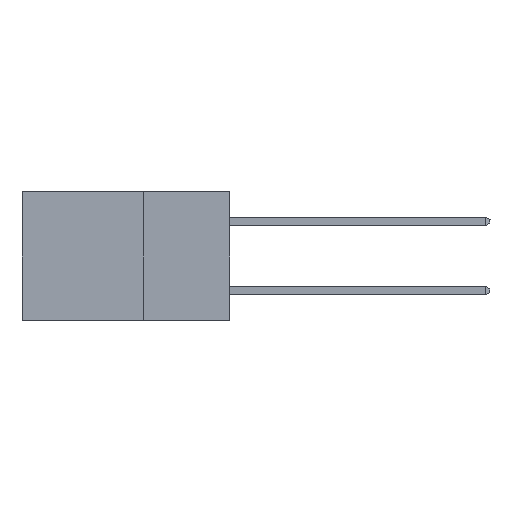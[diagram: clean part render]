
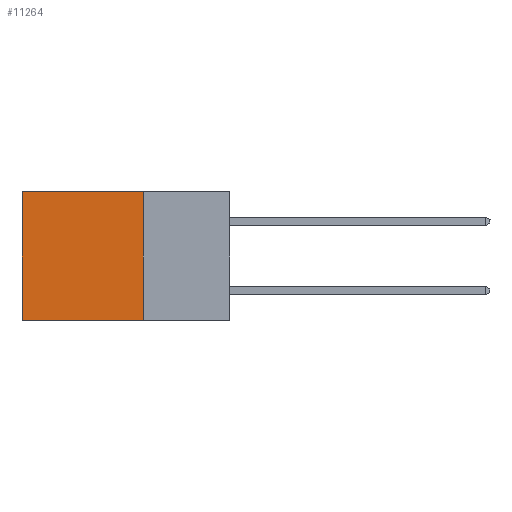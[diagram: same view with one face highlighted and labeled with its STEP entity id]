
A CAD part, left-side view. The second image highlights one B-rep face of the part: STEP entity #11264.
In plain terms, the highlighted planar face has unit normal (-1, 0, 0).
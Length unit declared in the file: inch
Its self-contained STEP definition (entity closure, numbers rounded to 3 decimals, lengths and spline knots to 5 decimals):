
#249 = CARTESIAN_POINT ( 'NONE',  ( 0.2615, 0.6, -0.37 ) ) ;
#918 = LINE ( 'NONE', #2823, #9138 ) ;
#1478 = CARTESIAN_POINT ( 'NONE',  ( 0.2615, 0.25, -0.37 ) ) ;
#1651 = DIRECTION ( 'NONE',  ( 0., 0., -1. ) ) ;
#2025 = VERTEX_POINT ( 'NONE', #4107 ) ;
#2049 = VECTOR ( 'NONE', #11312, 39.37008 ) ;
#2222 = EDGE_CURVE ( 'NONE', #2025, #11025, #11694, .T. ) ;
#2525 = EDGE_CURVE ( 'NONE', #6565, #2025, #3249, .T. ) ;
#2746 = ORIENTED_EDGE ( 'NONE', *, *, #4701, .F. ) ;
#2823 = CARTESIAN_POINT ( 'NONE',  ( 0.2615, 0.25, -0.37 ) ) ;
#2990 = ORIENTED_EDGE ( 'NONE', *, *, #11707, .F. ) ;
#3249 = LINE ( 'NONE', #8726, #2049 ) ;
#3406 = VECTOR ( 'NONE', #7565, 39.37008 ) ;
#3490 = DIRECTION ( 'NONE',  ( 1., 0., 0. ) ) ;
#4107 = CARTESIAN_POINT ( 'NONE',  ( 0.2615, 0.6, 0. ) ) ;
#4701 = EDGE_CURVE ( 'NONE', #6565, #5254, #9544, .T. ) ;
#4747 = EDGE_LOOP ( 'NONE', ( #6612, #2990, #2746, #5956 ) ) ;
#5254 = VERTEX_POINT ( 'NONE', #1478 ) ;
#5823 = CARTESIAN_POINT ( 'NONE',  ( 0.2615, 0.25, -0.37 ) ) ;
#5956 = ORIENTED_EDGE ( 'NONE', *, *, #2525, .T. ) ;
#6172 = CARTESIAN_POINT ( 'NONE',  ( 0.2615, 0.6, -0.37 ) ) ;
#6565 = VERTEX_POINT ( 'NONE', #8950 ) ;
#6612 = ORIENTED_EDGE ( 'NONE', *, *, #2222, .T. ) ;
#7565 = DIRECTION ( 'NONE',  ( 0., 0., -1. ) ) ;
#8726 = CARTESIAN_POINT ( 'NONE',  ( 0.2615, 0.25, 0. ) ) ;
#8893 = FACE_OUTER_BOUND ( 'NONE', #4747, .T. ) ;
#8950 = CARTESIAN_POINT ( 'NONE',  ( 0.2615, 0.25, 0. ) ) ;
#9138 = VECTOR ( 'NONE', #10096, 39.37008 ) ;
#9544 = LINE ( 'NONE', #11224, #3406 ) ;
#9623 = VECTOR ( 'NONE', #1651, 39.37008 ) ;
#9904 = AXIS2_PLACEMENT_3D ( 'NONE', #5823, #3490, #10770 ) ;
#10096 = DIRECTION ( 'NONE',  ( 0., 1., 0. ) ) ;
#10770 = DIRECTION ( 'NONE',  ( 0., 0., -1. ) ) ;
#11025 = VERTEX_POINT ( 'NONE', #249 ) ;
#11224 = CARTESIAN_POINT ( 'NONE',  ( 0.2615, 0.25, -0.37 ) ) ;
#11264 = ADVANCED_FACE ( 'NONE', ( #8893 ), #11685, .F. ) ;
#11312 = DIRECTION ( 'NONE',  ( 0., 1., 0. ) ) ;
#11685 = PLANE ( 'NONE',  #9904 ) ;
#11694 = LINE ( 'NONE', #6172, #9623 ) ;
#11707 = EDGE_CURVE ( 'NONE', #5254, #11025, #918, .T. ) ;
